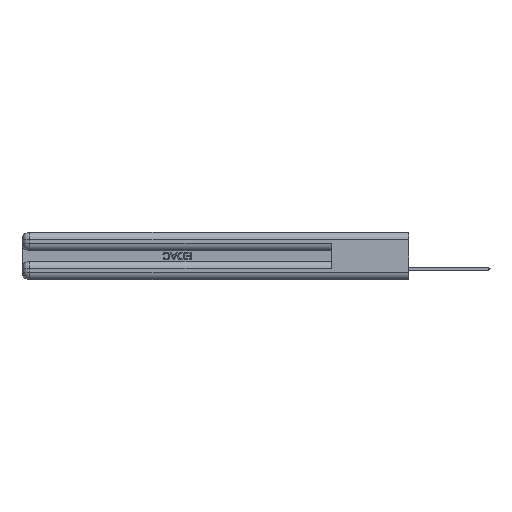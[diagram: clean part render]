
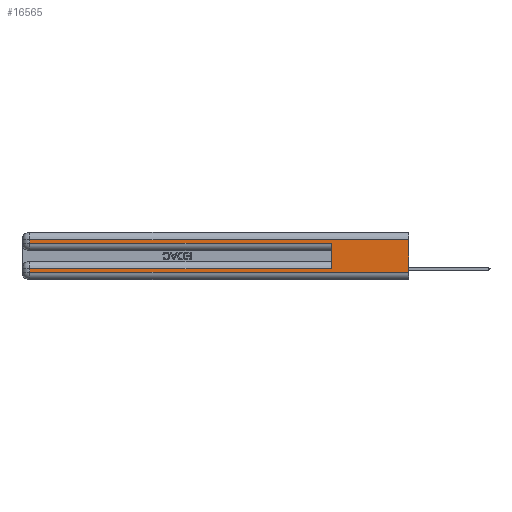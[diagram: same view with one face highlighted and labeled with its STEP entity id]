
A CAD part, left-side view. The second image highlights one B-rep face of the part: STEP entity #16565.
In plain terms, the highlighted planar face has unit normal (-1, 0, 0).
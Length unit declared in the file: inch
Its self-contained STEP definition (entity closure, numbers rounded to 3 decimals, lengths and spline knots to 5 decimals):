
#65 = VECTOR ( 'NONE', #26517, 39.37008 ) ;
#1163 = CARTESIAN_POINT ( 'NONE',  ( 0., 0., 0.285 ) ) ;
#1221 = CARTESIAN_POINT ( 'NONE',  ( 0., 0., 0.06 ) ) ;
#2212 = CARTESIAN_POINT ( 'NONE',  ( 0., 0., 0.31 ) ) ;
#2918 = VERTEX_POINT ( 'NONE', #8673 ) ;
#7070 = DIRECTION ( 'NONE',  ( 0., 0., -1. ) ) ;
#7429 = VECTOR ( 'NONE', #44247, 39.37008 ) ;
#7952 = LINE ( 'NONE', #12118, #10547 ) ;
#8673 = CARTESIAN_POINT ( 'NONE',  ( 0., 2.94, 0.085 ) ) ;
#9560 = DIRECTION ( 'NONE',  ( 0., 1., 0. ) ) ;
#10293 = LINE ( 'NONE', #1221, #22814 ) ;
#10547 = VECTOR ( 'NONE', #34204, 39.37008 ) ;
#12118 = CARTESIAN_POINT ( 'NONE',  ( 0., 0.6, 0.145 ) ) ;
#12938 = CARTESIAN_POINT ( 'NONE',  ( 0., 0., 0.085 ) ) ;
#13314 = EDGE_CURVE ( 'NONE', #20987, #2918, #27583, .T. ) ;
#13542 = LINE ( 'NONE', #1163, #40721 ) ;
#14232 = ORIENTED_EDGE ( 'NONE', *, *, #27043, .T. ) ;
#16565 = ADVANCED_FACE ( 'NONE', ( #21244 ), #33717, .F. ) ;
#18261 = CARTESIAN_POINT ( 'NONE',  ( 0., 0., 0.37 ) ) ;
#18415 = VECTOR ( 'NONE', #9560, 39.37008 ) ;
#20987 = VERTEX_POINT ( 'NONE', #34725 ) ;
#21244 = FACE_OUTER_BOUND ( 'NONE', #31374, .T. ) ;
#21767 = VERTEX_POINT ( 'NONE', #35219 ) ;
#21837 = EDGE_CURVE ( 'NONE', #36928, #53687, #38380, .T. ) ;
#22250 = VECTOR ( 'NONE', #50835, 39.37008 ) ;
#22439 = VERTEX_POINT ( 'NONE', #49173 ) ;
#22814 = VECTOR ( 'NONE', #25989, 39.37008 ) ;
#23212 = ORIENTED_EDGE ( 'NONE', *, *, #47039, .T. ) ;
#23895 = LINE ( 'NONE', #44643, #7429 ) ;
#25758 = VECTOR ( 'NONE', #7070, 39.37008 ) ;
#25989 = DIRECTION ( 'NONE',  ( 0., -1., 0. ) ) ;
#26517 = DIRECTION ( 'NONE',  ( 0., 0., -1. ) ) ;
#27043 = EDGE_CURVE ( 'NONE', #53687, #21767, #13542, .T. ) ;
#27583 = LINE ( 'NONE', #12938, #22250 ) ;
#28994 = ORIENTED_EDGE ( 'NONE', *, *, #53141, .F. ) ;
#29883 = ORIENTED_EDGE ( 'NONE', *, *, #21837, .T. ) ;
#30298 = CARTESIAN_POINT ( 'NONE',  ( 0., 2.94, 0.06 ) ) ;
#30519 = EDGE_CURVE ( 'NONE', #41176, #36928, #42343, .T. ) ;
#31374 = EDGE_LOOP ( 'NONE', ( #28994, #40827, #29883, #14232, #39068, #37113, #41866, #23212 ) ) ;
#33717 = PLANE ( 'NONE',  #41667 ) ;
#34204 = DIRECTION ( 'NONE',  ( 0., 0., 1. ) ) ;
#34725 = CARTESIAN_POINT ( 'NONE',  ( 0., 0.6, 0.085 ) ) ;
#35219 = CARTESIAN_POINT ( 'NONE',  ( 0., 0.6, 0.285 ) ) ;
#35924 = CARTESIAN_POINT ( 'NONE',  ( 0., 2.94, 0.31 ) ) ;
#36928 = VERTEX_POINT ( 'NONE', #35924 ) ;
#37113 = ORIENTED_EDGE ( 'NONE', *, *, #13314, .T. ) ;
#37994 = DIRECTION ( 'NONE',  ( 0., 0., -1. ) ) ;
#38380 = LINE ( 'NONE', #48576, #25758 ) ;
#39068 = ORIENTED_EDGE ( 'NONE', *, *, #54358, .F. ) ;
#40721 = VECTOR ( 'NONE', #43543, 39.37008 ) ;
#40827 = ORIENTED_EDGE ( 'NONE', *, *, #30519, .T. ) ;
#41176 = VERTEX_POINT ( 'NONE', #2212 ) ;
#41667 = AXIS2_PLACEMENT_3D ( 'NONE', #42957, #51390, #37994 ) ;
#41866 = ORIENTED_EDGE ( 'NONE', *, *, #52589, .T. ) ;
#42343 = LINE ( 'NONE', #46756, #18415 ) ;
#42957 = CARTESIAN_POINT ( 'NONE',  ( 0., 0., 0.37 ) ) ;
#43543 = DIRECTION ( 'NONE',  ( 0., -1., 0. ) ) ;
#44247 = DIRECTION ( 'NONE',  ( 0., 0., -1. ) ) ;
#44643 = CARTESIAN_POINT ( 'NONE',  ( 0., 2.94, 0.37 ) ) ;
#46756 = CARTESIAN_POINT ( 'NONE',  ( 0., 0., 0.31 ) ) ;
#47039 = EDGE_CURVE ( 'NONE', #52360, #22439, #10293, .T. ) ;
#48576 = CARTESIAN_POINT ( 'NONE',  ( 0., 2.94, 0.37 ) ) ;
#49173 = CARTESIAN_POINT ( 'NONE',  ( 0., 0., 0.06 ) ) ;
#49496 = CARTESIAN_POINT ( 'NONE',  ( 0., 2.94, 0.285 ) ) ;
#50835 = DIRECTION ( 'NONE',  ( 0., 1., 0. ) ) ;
#51390 = DIRECTION ( 'NONE',  ( 1., 0., 0. ) ) ;
#51566 = LINE ( 'NONE', #18261, #65 ) ;
#52360 = VERTEX_POINT ( 'NONE', #30298 ) ;
#52589 = EDGE_CURVE ( 'NONE', #2918, #52360, #23895, .T. ) ;
#53141 = EDGE_CURVE ( 'NONE', #41176, #22439, #51566, .T. ) ;
#53687 = VERTEX_POINT ( 'NONE', #49496 ) ;
#54358 = EDGE_CURVE ( 'NONE', #20987, #21767, #7952, .T. ) ;
